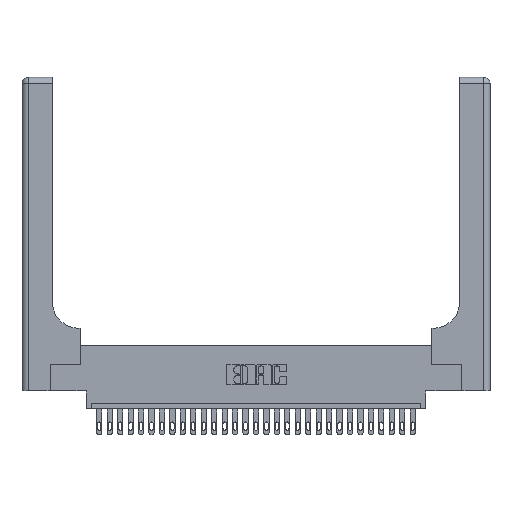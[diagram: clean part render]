
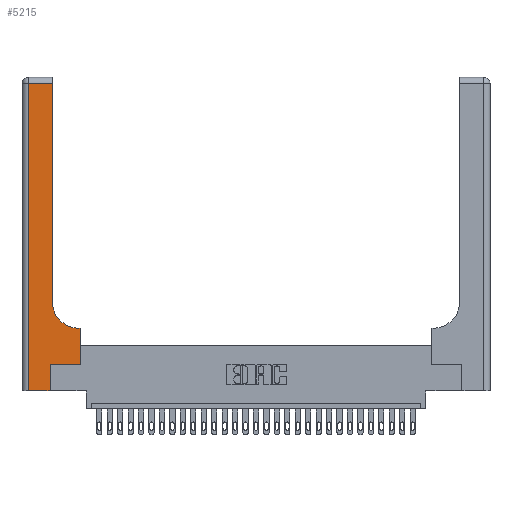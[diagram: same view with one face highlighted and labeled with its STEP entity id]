
A CAD part, top view. The second image highlights one B-rep face of the part: STEP entity #5215.
In plain terms, the highlighted planar face has unit normal (0, 0, 1).
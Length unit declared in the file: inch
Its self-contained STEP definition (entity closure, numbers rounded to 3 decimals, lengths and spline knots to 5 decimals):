
#69 = CARTESIAN_POINT ( 'NONE',  ( 0.269, 0., 0.37 ) ) ;
#235 = VERTEX_POINT ( 'NONE', #20044 ) ;
#1362 = EDGE_CURVE ( 'NONE', #235, #23668, #4435, .T. ) ;
#2441 = LINE ( 'NONE', #16533, #16211 ) ;
#2565 = VERTEX_POINT ( 'NONE', #5615 ) ;
#2875 = CARTESIAN_POINT ( 'NONE',  ( 0., 0., 0.37 ) ) ;
#2999 = DIRECTION ( 'NONE',  ( 0., -1., 0. ) ) ;
#3053 = CARTESIAN_POINT ( 'NONE',  ( 0.5585, 0.25, 0.37 ) ) ;
#3360 = CARTESIAN_POINT ( 'NONE',  ( 0.2915, 0.85, 0.37 ) ) ;
#3523 = DIRECTION ( 'NONE',  ( 0., 1., 0. ) ) ;
#4069 = AXIS2_PLACEMENT_3D ( 'NONE', #9942, #11902, #16488 ) ;
#4191 = VECTOR ( 'NONE', #3523, 39.37008 ) ;
#4435 = LINE ( 'NONE', #69, #24712 ) ;
#4445 = EDGE_CURVE ( 'NONE', #18582, #21566, #2441, .T. ) ;
#4865 = VECTOR ( 'NONE', #2999, 39.37008 ) ;
#5018 = EDGE_CURVE ( 'NONE', #26481, #25834, #5315, .T. ) ;
#5215 = ADVANCED_FACE ( 'NONE', ( #18360 ), #7237, .F. ) ;
#5315 = CIRCLE ( 'NONE', #20372, 0.25 ) ;
#5495 = EDGE_CURVE ( 'NONE', #25834, #18582, #19431, .T. ) ;
#5615 = CARTESIAN_POINT ( 'NONE',  ( 0.06, 0., 0.37 ) ) ;
#6188 = EDGE_CURVE ( 'NONE', #2565, #235, #22267, .T. ) ;
#7237 = PLANE ( 'NONE',  #4069 ) ;
#7885 = CARTESIAN_POINT ( 'NONE',  ( 0.5585, 0.6, 0.37 ) ) ;
#8200 = DIRECTION ( 'NONE',  ( 1., 0., 0. ) ) ;
#8237 = EDGE_CURVE ( 'NONE', #23664, #25702, #29929, .T. ) ;
#8628 = DIRECTION ( 'NONE',  ( -1., 0., 0. ) ) ;
#9024 = DIRECTION ( 'NONE',  ( 1., 0., 0. ) ) ;
#9512 = EDGE_CURVE ( 'NONE', #23668, #23664, #22623, .T. ) ;
#9691 = ORIENTED_EDGE ( 'NONE', *, *, #8237, .T. ) ;
#9942 = CARTESIAN_POINT ( 'NONE',  ( 0., 3., 0.37 ) ) ;
#11686 = ORIENTED_EDGE ( 'NONE', *, *, #13883, .T. ) ;
#11902 = DIRECTION ( 'NONE',  ( 0., 0., -1. ) ) ;
#12250 = ORIENTED_EDGE ( 'NONE', *, *, #9512, .T. ) ;
#13883 = EDGE_CURVE ( 'NONE', #21566, #2565, #20105, .T. ) ;
#14369 = EDGE_LOOP ( 'NONE', ( #15168, #16697, #11686, #19018, #20597, #12250, #9691, #24225, #16251 ) ) ;
#15168 = ORIENTED_EDGE ( 'NONE', *, *, #5495, .T. ) ;
#15599 = DIRECTION ( 'NONE',  ( 1., 0., 0. ) ) ;
#16211 = VECTOR ( 'NONE', #20836, 39.37008 ) ;
#16251 = ORIENTED_EDGE ( 'NONE', *, *, #5018, .T. ) ;
#16284 = DIRECTION ( 'NONE',  ( 0., 1., 0. ) ) ;
#16445 = VECTOR ( 'NONE', #9024, 39.37008 ) ;
#16488 = DIRECTION ( 'NONE',  ( -1., 0., 0. ) ) ;
#16533 = CARTESIAN_POINT ( 'NONE',  ( 0., 2.94, 0.37 ) ) ;
#16697 = ORIENTED_EDGE ( 'NONE', *, *, #4445, .T. ) ;
#17398 = CARTESIAN_POINT ( 'NONE',  ( 0.2915, 3., 0.37 ) ) ;
#17728 = CARTESIAN_POINT ( 'NONE',  ( 0.5415, 0.6, 0.37 ) ) ;
#17752 = DIRECTION ( 'NONE',  ( 0., 1., 0. ) ) ;
#18360 = FACE_OUTER_BOUND ( 'NONE', #14369, .T. ) ;
#18582 = VERTEX_POINT ( 'NONE', #22699 ) ;
#18596 = CARTESIAN_POINT ( 'NONE',  ( 0.06, 2.94, 0.37 ) ) ;
#19018 = ORIENTED_EDGE ( 'NONE', *, *, #6188, .T. ) ;
#19020 = VECTOR ( 'NONE', #8628, 39.37008 ) ;
#19431 = LINE ( 'NONE', #17398, #4191 ) ;
#20044 = CARTESIAN_POINT ( 'NONE',  ( 0.269, 0., 0.37 ) ) ;
#20105 = LINE ( 'NONE', #28650, #4865 ) ;
#20372 = AXIS2_PLACEMENT_3D ( 'NONE', #25058, #27170, #15599 ) ;
#20597 = ORIENTED_EDGE ( 'NONE', *, *, #1362, .T. ) ;
#20836 = DIRECTION ( 'NONE',  ( -1., 0., 0. ) ) ;
#21566 = VERTEX_POINT ( 'NONE', #18596 ) ;
#22267 = LINE ( 'NONE', #2875, #26970 ) ;
#22623 = LINE ( 'NONE', #30070, #16445 ) ;
#22699 = CARTESIAN_POINT ( 'NONE',  ( 0.2915, 2.94, 0.37 ) ) ;
#23664 = VERTEX_POINT ( 'NONE', #29221 ) ;
#23668 = VERTEX_POINT ( 'NONE', #28913 ) ;
#24225 = ORIENTED_EDGE ( 'NONE', *, *, #25348, .T. ) ;
#24699 = CARTESIAN_POINT ( 'NONE',  ( 0.2915, 0.6, 0.37 ) ) ;
#24712 = VECTOR ( 'NONE', #16284, 39.37008 ) ;
#24832 = VECTOR ( 'NONE', #17752, 39.37008 ) ;
#25058 = CARTESIAN_POINT ( 'NONE',  ( 0.5415, 0.85, 0.37 ) ) ;
#25198 = LINE ( 'NONE', #24699, #19020 ) ;
#25348 = EDGE_CURVE ( 'NONE', #25702, #26481, #25198, .T. ) ;
#25702 = VERTEX_POINT ( 'NONE', #7885 ) ;
#25834 = VERTEX_POINT ( 'NONE', #3360 ) ;
#26481 = VERTEX_POINT ( 'NONE', #17728 ) ;
#26970 = VECTOR ( 'NONE', #8200, 39.37008 ) ;
#27170 = DIRECTION ( 'NONE',  ( 0., 0., -1. ) ) ;
#28650 = CARTESIAN_POINT ( 'NONE',  ( 0.06, 3., 0.37 ) ) ;
#28913 = CARTESIAN_POINT ( 'NONE',  ( 0.269, 0.25, 0.37 ) ) ;
#29221 = CARTESIAN_POINT ( 'NONE',  ( 0.5585, 0.25, 0.37 ) ) ;
#29929 = LINE ( 'NONE', #3053, #24832 ) ;
#30070 = CARTESIAN_POINT ( 'NONE',  ( 0.269, 0.25, 0.37 ) ) ;
